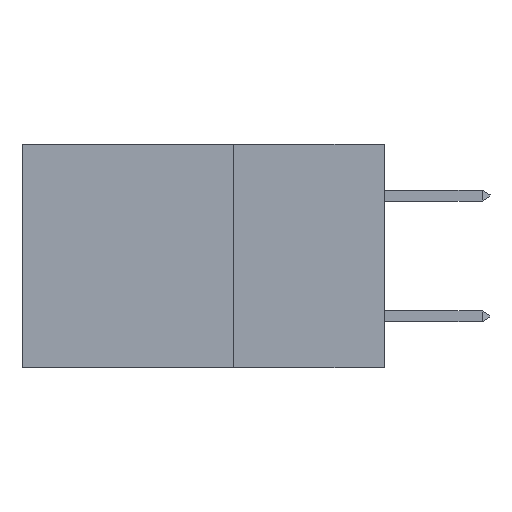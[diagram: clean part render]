
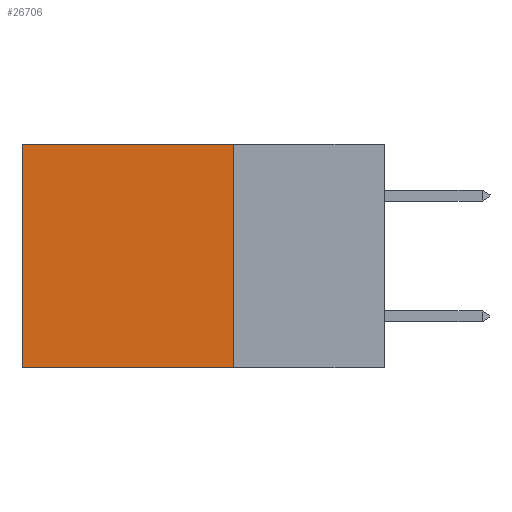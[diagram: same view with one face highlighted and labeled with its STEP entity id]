
A CAD part, left-side view. The second image highlights one B-rep face of the part: STEP entity #26706.
In plain terms, the highlighted planar face has unit normal (-1, 0, 0).
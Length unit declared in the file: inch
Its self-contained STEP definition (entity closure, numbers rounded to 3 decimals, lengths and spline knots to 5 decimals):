
#479 = LINE ( 'NONE', #23699, #30987 ) ;
#1085 = AXIS2_PLACEMENT_3D ( 'NONE', #32709, #38460, #14662 ) ;
#1202 = ORIENTED_EDGE ( 'NONE', *, *, #37059, .F. ) ;
#2663 = LINE ( 'NONE', #31133, #13495 ) ;
#4905 = ORIENTED_EDGE ( 'NONE', *, *, #7524, .F. ) ;
#7524 = EDGE_CURVE ( 'NONE', #16793, #22003, #14113, .T. ) ;
#7972 = LINE ( 'NONE', #12759, #9392 ) ;
#9392 = VECTOR ( 'NONE', #15773, 39.37008 ) ;
#9894 = DIRECTION ( 'NONE',  ( 0., 1., 0. ) ) ;
#10334 = DIRECTION ( 'NONE',  ( 0., 1., 0. ) ) ;
#12759 = CARTESIAN_POINT ( 'NONE',  ( 0.2875, 0.6, 0. ) ) ;
#12894 = CARTESIAN_POINT ( 'NONE',  ( 0.2875, 0.25, -0.37 ) ) ;
#13495 = VECTOR ( 'NONE', #10334, 39.37008 ) ;
#14113 = LINE ( 'NONE', #21565, #28163 ) ;
#14242 = EDGE_CURVE ( 'NONE', #19648, #21693, #7972, .T. ) ;
#14662 = DIRECTION ( 'NONE',  ( 0., 0., -1. ) ) ;
#15773 = DIRECTION ( 'NONE',  ( 0., 0., -1. ) ) ;
#15823 = DIRECTION ( 'NONE',  ( 0., 0., -1. ) ) ;
#16793 = VERTEX_POINT ( 'NONE', #26999 ) ;
#18806 = FACE_OUTER_BOUND ( 'NONE', #37459, .T. ) ;
#19648 = VERTEX_POINT ( 'NONE', #35309 ) ;
#21565 = CARTESIAN_POINT ( 'NONE',  ( 0.2875, 0.25, 0. ) ) ;
#21693 = VERTEX_POINT ( 'NONE', #35302 ) ;
#22003 = VERTEX_POINT ( 'NONE', #12894 ) ;
#22052 = EDGE_CURVE ( 'NONE', #16793, #19648, #479, .T. ) ;
#23412 = ORIENTED_EDGE ( 'NONE', *, *, #14242, .T. ) ;
#23699 = CARTESIAN_POINT ( 'NONE',  ( 0.2875, 0.25, 0. ) ) ;
#26706 = ADVANCED_FACE ( 'NONE', ( #18806 ), #35214, .F. ) ;
#26999 = CARTESIAN_POINT ( 'NONE',  ( 0.2875, 0.25, 0. ) ) ;
#28163 = VECTOR ( 'NONE', #15823, 39.37008 ) ;
#30142 = ORIENTED_EDGE ( 'NONE', *, *, #22052, .T. ) ;
#30987 = VECTOR ( 'NONE', #9894, 39.37008 ) ;
#31133 = CARTESIAN_POINT ( 'NONE',  ( 0.2875, 0.25, -0.37 ) ) ;
#32709 = CARTESIAN_POINT ( 'NONE',  ( 0.2875, 0.25, 0. ) ) ;
#35214 = PLANE ( 'NONE',  #1085 ) ;
#35302 = CARTESIAN_POINT ( 'NONE',  ( 0.2875, 0.6, -0.37 ) ) ;
#35309 = CARTESIAN_POINT ( 'NONE',  ( 0.2875, 0.6, 0. ) ) ;
#37059 = EDGE_CURVE ( 'NONE', #22003, #21693, #2663, .T. ) ;
#37459 = EDGE_LOOP ( 'NONE', ( #23412, #1202, #4905, #30142 ) ) ;
#38460 = DIRECTION ( 'NONE',  ( 1., 0., 0. ) ) ;
